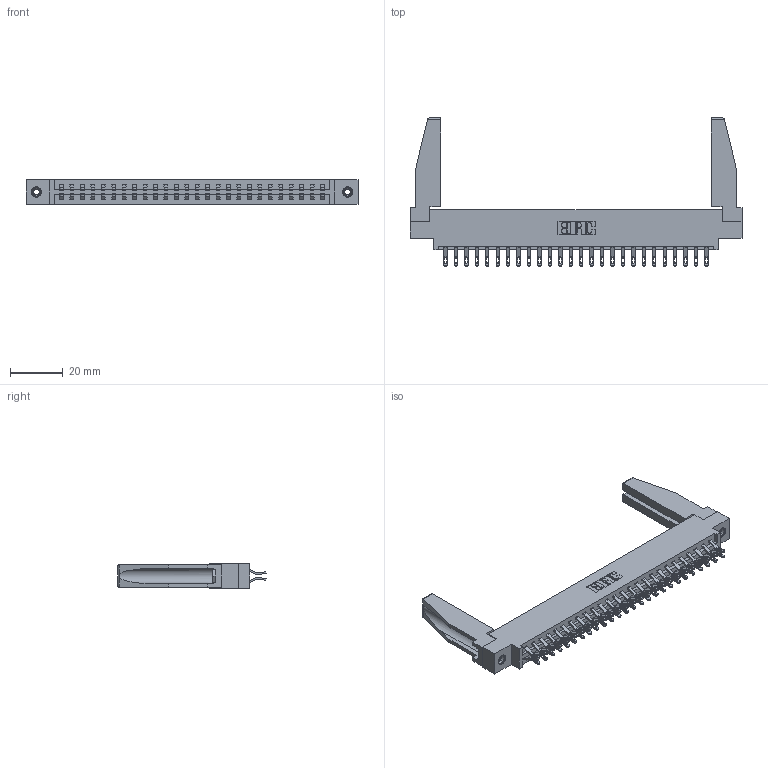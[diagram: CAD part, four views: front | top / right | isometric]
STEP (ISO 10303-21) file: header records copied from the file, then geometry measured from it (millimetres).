
FILE_DESCRIPTION (( 'STEP AP203' ), '1' );
FILE_NAME ('387-052-555-878.STEP', '2019-10-19T03:46:17', ( '' ), ( '' ), 'SwSTEP 2.0', 'SolidWorks 2016', '' );
FILE_SCHEMA (( 'CONFIG_CONTROL_DESIGN' ));
Length unit declared in the file: inch
Products named in the file (5): 345-250-001_345-250-001-102; 345-292-001_555 Tail; 387-052-555-878; 307-220-078; 337 Part_0.170 Offset - 0.156 Dia-TI
Assembly tree (57 placements, depth 2):
  387-052-555-878
    337 Part_0.170 Offset - 0.156 Dia-TI
    345-292-001_555 Tail  x52
    345-250-001_345-250-001-102  x2
    307-220-078  x2
Bounding box: 126.03 x 56.27 x 9.4 mm (x, y, z)
Volume: 17096.2 mm3; surface area: 19164.1 mm2
Topology: 57 solids, 57 shells, 3368 faces, 10481 edges, 6978 vertices
Faces by surface type: plane 2030, cylinder 1322, cone 12, torus 4
Entity records: 25126 total; most frequent: CARTESIAN_POINT 4282, ORIENTED_EDGE 4144, DIRECTION 3648, EDGE_CURVE 2072, LINE 1886, VECTOR 1886, VERTEX_POINT 1376, AXIS2_PLACEMENT_3D 881
